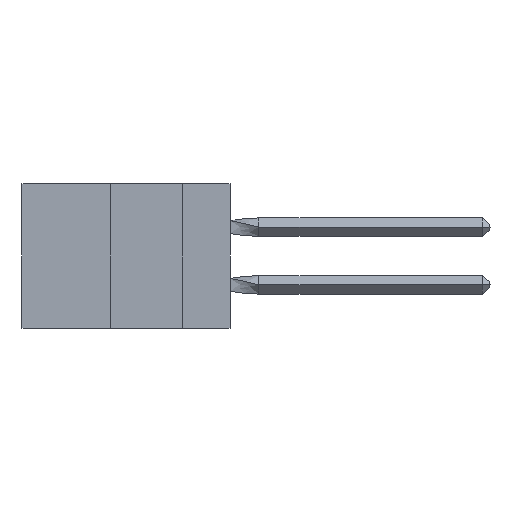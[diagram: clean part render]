
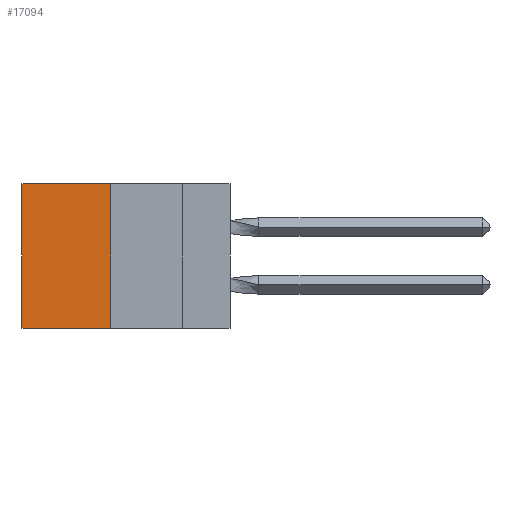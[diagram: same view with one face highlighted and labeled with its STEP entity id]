
A CAD part, left-side view. The second image highlights one B-rep face of the part: STEP entity #17094.
In plain terms, the highlighted planar face has unit normal (-1, 0, 0).
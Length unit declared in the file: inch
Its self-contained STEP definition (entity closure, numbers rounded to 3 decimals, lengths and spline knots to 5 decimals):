
#571 = ORIENTED_EDGE ( 'NONE', *, *, #14903, .T. ) ;
#924 = VERTEX_POINT ( 'NONE', #21189 ) ;
#1152 = DIRECTION ( 'NONE',  ( 0., 1., 0. ) ) ;
#1301 = LINE ( 'NONE', #9396, #2124 ) ;
#1486 = DIRECTION ( 'NONE',  ( 0., 0., -1. ) ) ;
#1759 = EDGE_CURVE ( 'NONE', #924, #13205, #19696, .T. ) ;
#2124 = VECTOR ( 'NONE', #15452, 39.37008 ) ;
#2241 = DIRECTION ( 'NONE',  ( 0., 0., -1. ) ) ;
#4925 = VECTOR ( 'NONE', #1152, 39.37008 ) ;
#6874 = CARTESIAN_POINT ( 'NONE',  ( 0.305, 0.413, -0.5 ) ) ;
#7165 = VERTEX_POINT ( 'NONE', #15293 ) ;
#8159 = VECTOR ( 'NONE', #20595, 39.37008 ) ;
#8645 = ORIENTED_EDGE ( 'NONE', *, *, #1759, .F. ) ;
#8722 = CARTESIAN_POINT ( 'NONE',  ( 0.305, 0.413, -0.5 ) ) ;
#9396 = CARTESIAN_POINT ( 'NONE',  ( 0.305, 0.413, 0. ) ) ;
#9666 = LINE ( 'NONE', #20531, #4925 ) ;
#11023 = EDGE_CURVE ( 'NONE', #13205, #7165, #9666, .T. ) ;
#11326 = ORIENTED_EDGE ( 'NONE', *, *, #11023, .F. ) ;
#12110 = PLANE ( 'NONE',  #16039 ) ;
#13007 = CARTESIAN_POINT ( 'NONE',  ( 0.305, 0.72, -0.5 ) ) ;
#13205 = VERTEX_POINT ( 'NONE', #6874 ) ;
#13207 = EDGE_CURVE ( 'NONE', #924, #14606, #1301, .T. ) ;
#14208 = VECTOR ( 'NONE', #2241, 39.37008 ) ;
#14606 = VERTEX_POINT ( 'NONE', #22350 ) ;
#14903 = EDGE_CURVE ( 'NONE', #14606, #7165, #16929, .T. ) ;
#15293 = CARTESIAN_POINT ( 'NONE',  ( 0.305, 0.72, -0.5 ) ) ;
#15302 = CARTESIAN_POINT ( 'NONE',  ( 0.305, 0.413, -0.5 ) ) ;
#15452 = DIRECTION ( 'NONE',  ( 0., 1., 0. ) ) ;
#16039 = AXIS2_PLACEMENT_3D ( 'NONE', #8722, #22666, #1486 ) ;
#16929 = LINE ( 'NONE', #13007, #14208 ) ;
#17094 = ADVANCED_FACE ( 'NONE', ( #19464 ), #12110, .F. ) ;
#17340 = EDGE_LOOP ( 'NONE', ( #571, #11326, #8645, #21582 ) ) ;
#19464 = FACE_OUTER_BOUND ( 'NONE', #17340, .T. ) ;
#19696 = LINE ( 'NONE', #15302, #8159 ) ;
#20531 = CARTESIAN_POINT ( 'NONE',  ( 0.305, 0.413, -0.5 ) ) ;
#20595 = DIRECTION ( 'NONE',  ( 0., 0., -1. ) ) ;
#21189 = CARTESIAN_POINT ( 'NONE',  ( 0.305, 0.413, 0. ) ) ;
#21582 = ORIENTED_EDGE ( 'NONE', *, *, #13207, .T. ) ;
#22350 = CARTESIAN_POINT ( 'NONE',  ( 0.305, 0.72, 0. ) ) ;
#22666 = DIRECTION ( 'NONE',  ( 1., 0., 0. ) ) ;
